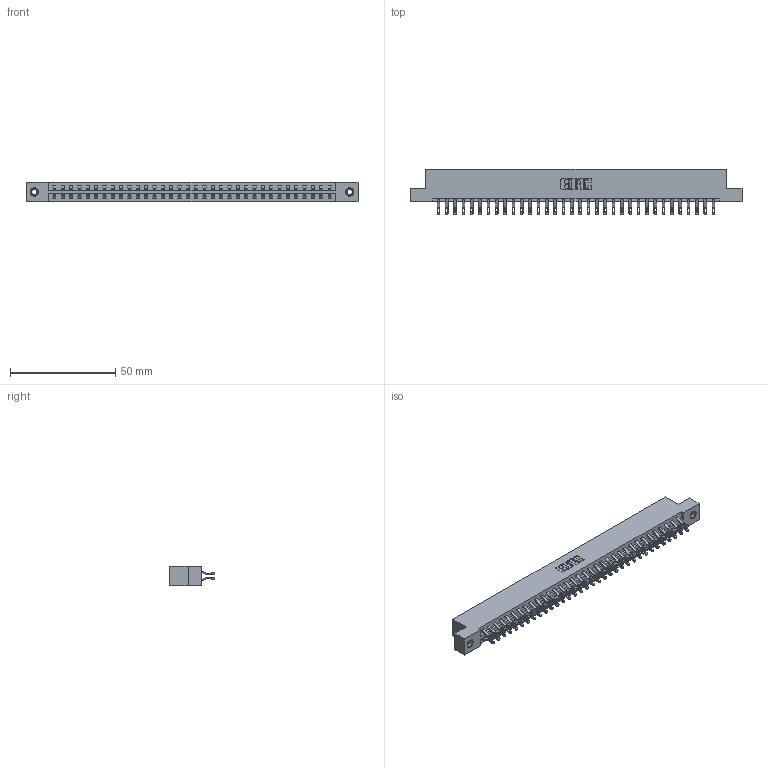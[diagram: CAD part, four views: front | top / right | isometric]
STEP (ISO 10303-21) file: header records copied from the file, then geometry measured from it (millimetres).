
FILE_DESCRIPTION (( 'STEP AP203' ), '1' );
FILE_NAME ('387-068-555-207.STEP', '2019-10-19T21:34:46', ( '' ), ( '' ), 'SwSTEP 2.0', 'SolidWorks 2016', '' );
FILE_SCHEMA (( 'CONFIG_CONTROL_DESIGN' ));
Length unit declared in the file: inch
Products named in the file (4): 337 Part_Flush Mounting Lugs - 0.156 Dia-TI; 387-068-555-207; 345-292-001_555 Tail; 345-250-001_345-250-005-103
Assembly tree (71 placements, depth 2):
  387-068-555-207
    337 Part_Flush Mounting Lugs - 0.156 Dia-TI
    345-292-001_555 Tail  x68
    345-250-001_345-250-005-103  x2
Bounding box: 157.73 x 21.47 x 9.4 mm (x, y, z)
Volume: 16700.5 mm3; surface area: 19581.5 mm2
Topology: 71 solids, 71 shells, 4254 faces, 13299 edges, 8858 vertices
Faces by surface type: plane 2550, cylinder 1688, cone 12, torus 4
Entity records: 28908 total; most frequent: CARTESIAN_POINT 4891, ORIENTED_EDGE 4790, DIRECTION 4177, EDGE_CURVE 2395, LINE 2227, VECTOR 2227, VERTEX_POINT 1592, AXIS2_PLACEMENT_3D 975
